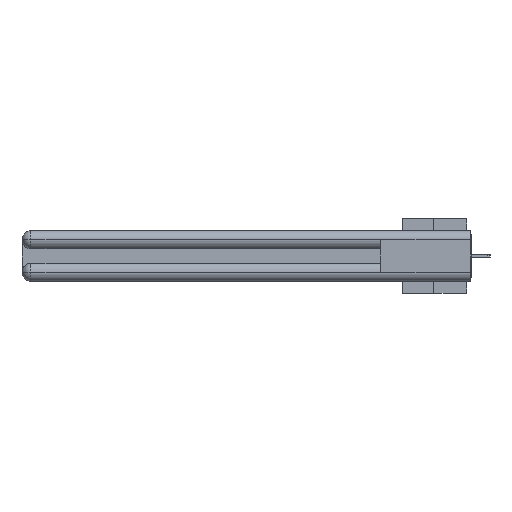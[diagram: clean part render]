
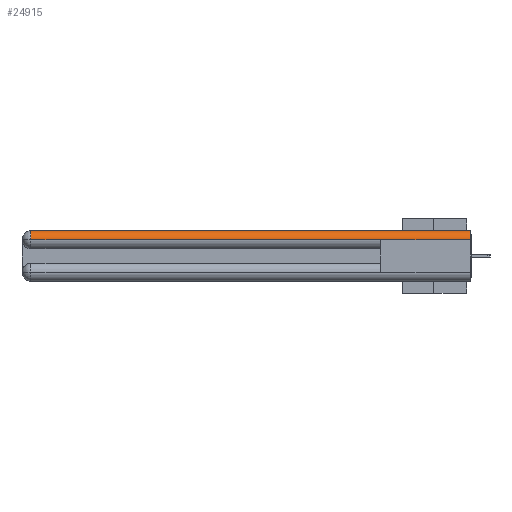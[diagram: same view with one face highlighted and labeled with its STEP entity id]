
A CAD part, left-side view. The second image highlights one B-rep face of the part: STEP entity #24915.
In plain terms, the highlighted cylindrical face has radius 1.562 mm (diameter 3.124 mm), a partial arc.
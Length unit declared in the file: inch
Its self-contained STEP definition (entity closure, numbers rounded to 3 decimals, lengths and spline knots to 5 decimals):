
#1241 = ORIENTED_EDGE ( 'NONE', *, *, #31508, .T. ) ;
#2349 = AXIS2_PLACEMENT_3D ( 'NONE', #9998, #23724, #9796 ) ;
#2681 = DIRECTION ( 'NONE',  ( 0., -1., 0. ) ) ;
#3715 = CARTESIAN_POINT ( 'NONE',  ( 0.0615, 0., -0.0615 ) ) ;
#5161 = VERTEX_POINT ( 'NONE', #36012 ) ;
#5714 = AXIS2_PLACEMENT_3D ( 'NONE', #21063, #23449, #17942 ) ;
#5836 = VERTEX_POINT ( 'NONE', #24782 ) ;
#6752 = CYLINDRICAL_SURFACE ( 'NONE', #5714, 0.0615 ) ;
#8636 = EDGE_LOOP ( 'NONE', ( #33777, #1241, #11364, #26792, #15565 ) ) ;
#8879 = DIRECTION ( 'NONE',  ( 0., -1., 0. ) ) ;
#9765 = EDGE_CURVE ( 'NONE', #13380, #5836, #22328, .T. ) ;
#9796 = DIRECTION ( 'NONE',  ( 0., 0., 1. ) ) ;
#9998 = CARTESIAN_POINT ( 'NONE',  ( 0.0615, 2.94, -0.0615 ) ) ;
#11176 = EDGE_CURVE ( 'NONE', #35658, #5161, #11911, .T. ) ;
#11364 = ORIENTED_EDGE ( 'NONE', *, *, #17989, .T. ) ;
#11911 = LINE ( 'NONE', #14838, #34258 ) ;
#12550 = CARTESIAN_POINT ( 'NONE',  ( 0.0615, 2.94, 0. ) ) ;
#13380 = VERTEX_POINT ( 'NONE', #18034 ) ;
#14414 = DIRECTION ( 'NONE',  ( 0., 1., 0. ) ) ;
#14838 = CARTESIAN_POINT ( 'NONE',  ( 0.0615, 0., 0. ) ) ;
#15565 = ORIENTED_EDGE ( 'NONE', *, *, #17231, .F. ) ;
#16611 = LINE ( 'NONE', #27768, #31569 ) ;
#17231 = EDGE_CURVE ( 'NONE', #5161, #13380, #24024, .T. ) ;
#17942 = DIRECTION ( 'NONE',  ( 0., 0., 1. ) ) ;
#17989 = EDGE_CURVE ( 'NONE', #21068, #5836, #16611, .T. ) ;
#18034 = CARTESIAN_POINT ( 'NONE',  ( 0., 0., -0.0615 ) ) ;
#19760 = CARTESIAN_POINT ( 'NONE',  ( 0., 3., -0.0615 ) ) ;
#20042 = DIRECTION ( 'NONE',  ( 1., 0., 0. ) ) ;
#21063 = CARTESIAN_POINT ( 'NONE',  ( 0.0615, 0., -0.0615 ) ) ;
#21068 = VERTEX_POINT ( 'NONE', #27578 ) ;
#21939 = VECTOR ( 'NONE', #14414, 39.37008 ) ;
#22215 = AXIS2_PLACEMENT_3D ( 'NONE', #3715, #8879, #20042 ) ;
#22328 = LINE ( 'NONE', #19760, #21939 ) ;
#23449 = DIRECTION ( 'NONE',  ( 0., 1., 0. ) ) ;
#23724 = DIRECTION ( 'NONE',  ( 0., -1., 0. ) ) ;
#23799 = FACE_OUTER_BOUND ( 'NONE', #8636, .T. ) ;
#24024 = CIRCLE ( 'NONE', #22215, 0.0615 ) ;
#24782 = CARTESIAN_POINT ( 'NONE',  ( 0., 0.6, -0.0615 ) ) ;
#24915 = ADVANCED_FACE ( 'NONE', ( #23799 ), #6752, .T. ) ;
#25709 = CIRCLE ( 'NONE', #2349, 0.0615 ) ;
#26792 = ORIENTED_EDGE ( 'NONE', *, *, #9765, .F. ) ;
#27578 = CARTESIAN_POINT ( 'NONE',  ( 0., 2.94, -0.0615 ) ) ;
#27768 = CARTESIAN_POINT ( 'NONE',  ( 0., 3., -0.0615 ) ) ;
#28932 = DIRECTION ( 'NONE',  ( 0., -1., 0. ) ) ;
#31508 = EDGE_CURVE ( 'NONE', #35658, #21068, #25709, .T. ) ;
#31569 = VECTOR ( 'NONE', #2681, 39.37008 ) ;
#33777 = ORIENTED_EDGE ( 'NONE', *, *, #11176, .F. ) ;
#34258 = VECTOR ( 'NONE', #28932, 39.37008 ) ;
#35658 = VERTEX_POINT ( 'NONE', #12550 ) ;
#36012 = CARTESIAN_POINT ( 'NONE',  ( 0.0615, 0., 0. ) ) ;
